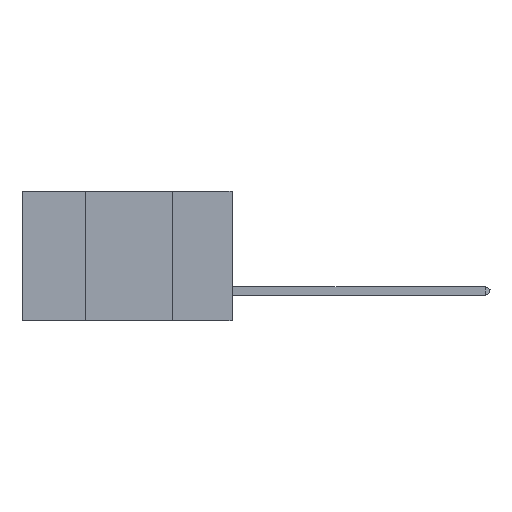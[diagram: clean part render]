
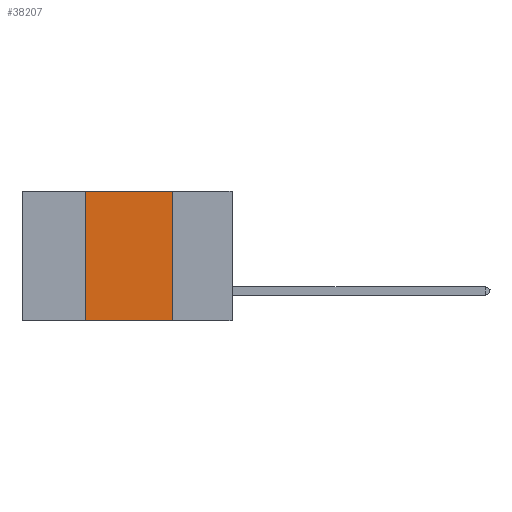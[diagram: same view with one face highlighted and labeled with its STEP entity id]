
A CAD part, left-side view. The second image highlights one B-rep face of the part: STEP entity #38207.
In plain terms, the highlighted planar face has unit normal (-1, 0, 0).
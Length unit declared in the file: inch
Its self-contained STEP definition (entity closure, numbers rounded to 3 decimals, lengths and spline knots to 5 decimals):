
#90 = ORIENTED_EDGE ( 'NONE', *, *, #972, .F. ) ;
#735 = VERTEX_POINT ( 'NONE', #5771 ) ;
#972 = EDGE_CURVE ( 'NONE', #35491, #14163, #24885, .T. ) ;
#981 = EDGE_CURVE ( 'NONE', #33300, #735, #19330, .T. ) ;
#1878 = CARTESIAN_POINT ( 'NONE',  ( 0., 0.6, -0.37 ) ) ;
#4825 = DIRECTION ( 'NONE',  ( 0., -1., 0. ) ) ;
#5771 = CARTESIAN_POINT ( 'NONE',  ( 0., 0.42, 0. ) ) ;
#6779 = LINE ( 'NONE', #11284, #36426 ) ;
#7618 = CARTESIAN_POINT ( 'NONE',  ( 0., 0.6, 0. ) ) ;
#7783 = DIRECTION ( 'NONE',  ( 0., -1., 0. ) ) ;
#9577 = VECTOR ( 'NONE', #19393, 39.37008 ) ;
#10997 = DIRECTION ( 'NONE',  ( 0., 0., -1. ) ) ;
#11284 = CARTESIAN_POINT ( 'NONE',  ( 0., 0.6, 0. ) ) ;
#11300 = FACE_OUTER_BOUND ( 'NONE', #27157, .T. ) ;
#12363 = VECTOR ( 'NONE', #16513, 39.37008 ) ;
#13794 = CARTESIAN_POINT ( 'NONE',  ( 0., 0.42, 0. ) ) ;
#14163 = VERTEX_POINT ( 'NONE', #30737 ) ;
#14354 = CARTESIAN_POINT ( 'NONE',  ( 0., 0.42, -0.37 ) ) ;
#16105 = EDGE_CURVE ( 'NONE', #33300, #14163, #17564, .T. ) ;
#16513 = DIRECTION ( 'NONE',  ( 0., 0., -1. ) ) ;
#17160 = ORIENTED_EDGE ( 'NONE', *, *, #24079, .F. ) ;
#17564 = LINE ( 'NONE', #1878, #36977 ) ;
#18446 = CARTESIAN_POINT ( 'NONE',  ( 0., 0.17, 0. ) ) ;
#19330 = LINE ( 'NONE', #13794, #9577 ) ;
#19393 = DIRECTION ( 'NONE',  ( 0., 0., 1. ) ) ;
#22545 = DIRECTION ( 'NONE',  ( 1., 0., 0. ) ) ;
#22799 = PLANE ( 'NONE',  #34183 ) ;
#24079 = EDGE_CURVE ( 'NONE', #735, #35491, #6779, .T. ) ;
#24885 = LINE ( 'NONE', #28262, #12363 ) ;
#27157 = EDGE_LOOP ( 'NONE', ( #90, #17160, #36474, #36389 ) ) ;
#28262 = CARTESIAN_POINT ( 'NONE',  ( 0., 0.17, 0. ) ) ;
#30737 = CARTESIAN_POINT ( 'NONE',  ( 0., 0.17, -0.37 ) ) ;
#33300 = VERTEX_POINT ( 'NONE', #14354 ) ;
#34183 = AXIS2_PLACEMENT_3D ( 'NONE', #7618, #22545, #10997 ) ;
#35491 = VERTEX_POINT ( 'NONE', #18446 ) ;
#36389 = ORIENTED_EDGE ( 'NONE', *, *, #16105, .T. ) ;
#36426 = VECTOR ( 'NONE', #7783, 39.37008 ) ;
#36474 = ORIENTED_EDGE ( 'NONE', *, *, #981, .F. ) ;
#36977 = VECTOR ( 'NONE', #4825, 39.37008 ) ;
#38207 = ADVANCED_FACE ( 'NONE', ( #11300 ), #22799, .F. ) ;
